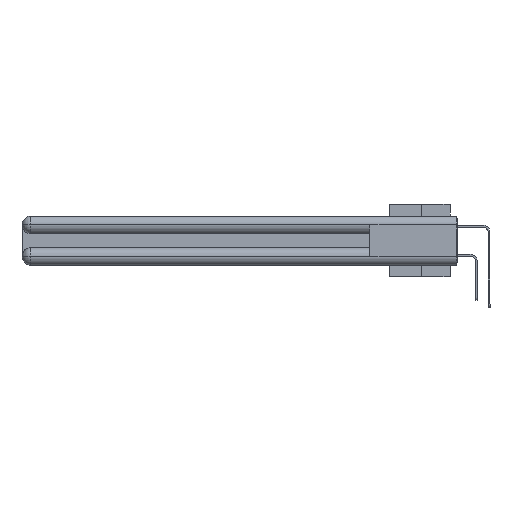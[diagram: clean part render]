
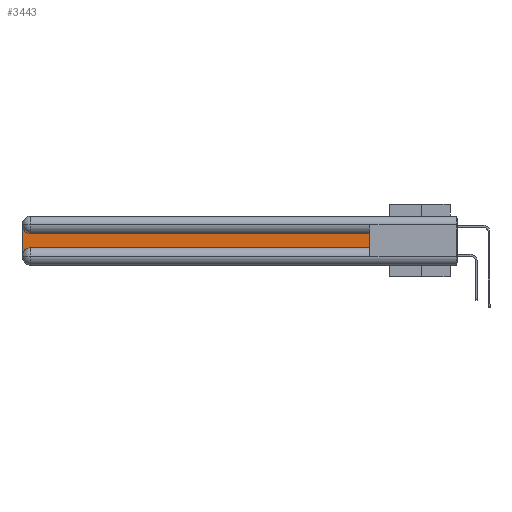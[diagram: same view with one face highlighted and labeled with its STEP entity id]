
A CAD part, left-side view. The second image highlights one B-rep face of the part: STEP entity #3443.
In plain terms, the highlighted planar face has unit normal (-1, 0, 0).
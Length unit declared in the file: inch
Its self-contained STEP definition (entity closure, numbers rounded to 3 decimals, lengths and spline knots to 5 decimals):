
#1191 = CARTESIAN_POINT ( 'NONE',  ( 0.075, 2.94, -0.2175 ) ) ;
#1335 = EDGE_CURVE ( 'NONE', #21050, #15700, #6705, .T. ) ;
#2045 = EDGE_CURVE ( 'NONE', #3530, #15222, #26159, .T. ) ;
#2508 = ORIENTED_EDGE ( 'NONE', *, *, #1335, .T. ) ;
#2572 = AXIS2_PLACEMENT_3D ( 'NONE', #9288, #19234, #27066 ) ;
#3382 = DIRECTION ( 'NONE',  ( 1., 0., 0. ) ) ;
#3443 = ADVANCED_FACE ( 'NONE', ( #27134 ), #29599, .F. ) ;
#3530 = VERTEX_POINT ( 'NONE', #17989 ) ;
#3571 = VECTOR ( 'NONE', #4262, 39.37008 ) ;
#3984 = ORIENTED_EDGE ( 'NONE', *, *, #2045, .T. ) ;
#4151 = VECTOR ( 'NONE', #15213, 39.37008 ) ;
#4262 = DIRECTION ( 'NONE',  ( 0., 1., 0. ) ) ;
#5012 = ORIENTED_EDGE ( 'NONE', *, *, #31390, .T. ) ;
#5706 = EDGE_CURVE ( 'NONE', #15700, #30877, #16685, .T. ) ;
#5985 = DIRECTION ( 'NONE',  ( 0., 0., -1. ) ) ;
#6705 = LINE ( 'NONE', #26615, #3571 ) ;
#7226 = DIRECTION ( 'NONE',  ( 0., 0., -1. ) ) ;
#8155 = ORIENTED_EDGE ( 'NONE', *, *, #30299, .T. ) ;
#8663 = CARTESIAN_POINT ( 'NONE',  ( 0.075, 0.6, -0.2175 ) ) ;
#9288 = CARTESIAN_POINT ( 'NONE',  ( 0.075, 2.94, -0.0625 ) ) ;
#10540 = DIRECTION ( 'NONE',  ( 0., -1., 0. ) ) ;
#11488 = EDGE_CURVE ( 'NONE', #15222, #13835, #15454, .T. ) ;
#11563 = CARTESIAN_POINT ( 'NONE',  ( 0.075, 3., -0.0625 ) ) ;
#12127 = AXIS2_PLACEMENT_3D ( 'NONE', #30318, #3382, #5985 ) ;
#13835 = VERTEX_POINT ( 'NONE', #8663 ) ;
#15213 = DIRECTION ( 'NONE',  ( 0., 0., 1. ) ) ;
#15222 = VERTEX_POINT ( 'NONE', #1191 ) ;
#15454 = LINE ( 'NONE', #30607, #20941 ) ;
#15700 = VERTEX_POINT ( 'NONE', #19777 ) ;
#16258 = CARTESIAN_POINT ( 'NONE',  ( 0.075, 3., -0.2175 ) ) ;
#16685 = CIRCLE ( 'NONE', #2572, 0.06 ) ;
#17989 = CARTESIAN_POINT ( 'NONE',  ( 0.075, 3., -0.2775 ) ) ;
#18313 = ORIENTED_EDGE ( 'NONE', *, *, #5706, .T. ) ;
#18424 = ORIENTED_EDGE ( 'NONE', *, *, #11488, .T. ) ;
#18691 = LINE ( 'NONE', #16258, #25569 ) ;
#19234 = DIRECTION ( 'NONE',  ( 1., 0., 0. ) ) ;
#19777 = CARTESIAN_POINT ( 'NONE',  ( 0.075, 2.94, -0.1225 ) ) ;
#20941 = VECTOR ( 'NONE', #10540, 39.37008 ) ;
#21050 = VERTEX_POINT ( 'NONE', #30108 ) ;
#21635 = DIRECTION ( 'NONE',  ( 0., 0., -1. ) ) ;
#22240 = CARTESIAN_POINT ( 'NONE',  ( 0.075, 0.6, -0.2175 ) ) ;
#24692 = CARTESIAN_POINT ( 'NONE',  ( 0.075, 3., -0.1225 ) ) ;
#25143 = LINE ( 'NONE', #22240, #4151 ) ;
#25569 = VECTOR ( 'NONE', #21635, 39.37008 ) ;
#25741 = AXIS2_PLACEMENT_3D ( 'NONE', #24692, #26978, #7226 ) ;
#26159 = CIRCLE ( 'NONE', #12127, 0.06 ) ;
#26615 = CARTESIAN_POINT ( 'NONE',  ( 0.075, 0.6, -0.1225 ) ) ;
#26978 = DIRECTION ( 'NONE',  ( 1., 0., 0. ) ) ;
#27066 = DIRECTION ( 'NONE',  ( 0., 0., -1. ) ) ;
#27134 = FACE_OUTER_BOUND ( 'NONE', #31204, .T. ) ;
#29599 = PLANE ( 'NONE',  #25741 ) ;
#30108 = CARTESIAN_POINT ( 'NONE',  ( 0.075, 0.6, -0.1225 ) ) ;
#30299 = EDGE_CURVE ( 'NONE', #13835, #21050, #25143, .T. ) ;
#30318 = CARTESIAN_POINT ( 'NONE',  ( 0.075, 2.94, -0.2775 ) ) ;
#30607 = CARTESIAN_POINT ( 'NONE',  ( 0.075, 0.6, -0.2175 ) ) ;
#30877 = VERTEX_POINT ( 'NONE', #11563 ) ;
#31204 = EDGE_LOOP ( 'NONE', ( #2508, #18313, #5012, #3984, #18424, #8155 ) ) ;
#31390 = EDGE_CURVE ( 'NONE', #30877, #3530, #18691, .T. ) ;
